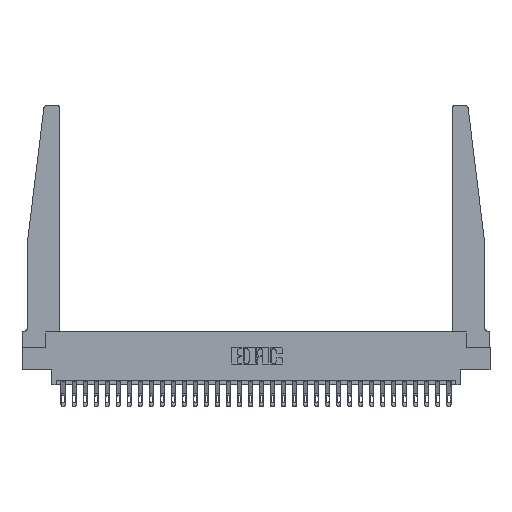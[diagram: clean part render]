
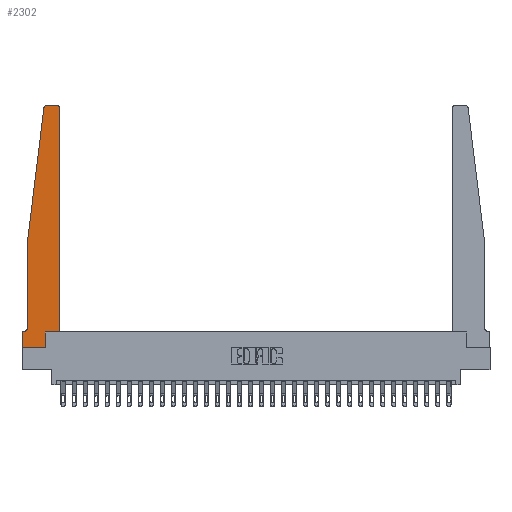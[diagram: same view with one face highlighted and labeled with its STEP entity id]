
A CAD part, top view. The second image highlights one B-rep face of the part: STEP entity #2302.
In plain terms, the highlighted planar face has unit normal (0, 0, 1).
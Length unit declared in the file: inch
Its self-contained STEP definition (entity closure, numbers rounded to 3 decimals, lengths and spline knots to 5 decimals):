
#673 = CARTESIAN_POINT ( 'NONE',  ( 0.24675, 2.72367, 0.37 ) ) ;
#2259 = CARTESIAN_POINT ( 'NONE',  ( 0.015, 0.2375, 0.37 ) ) ;
#2302 = ADVANCED_FACE ( 'NONE', ( #9067 ), #21267, .T. ) ;
#2728 = CARTESIAN_POINT ( 'NONE',  ( 0.425, 0.18, 0.37 ) ) ;
#3026 = LINE ( 'NONE', #15538, #26558 ) ;
#3067 = ORIENTED_EDGE ( 'NONE', *, *, #25364, .T. ) ;
#3499 = ORIENTED_EDGE ( 'NONE', *, *, #7070, .T. ) ;
#3506 = ORIENTED_EDGE ( 'NONE', *, *, #5088, .T. ) ;
#3825 = EDGE_CURVE ( 'NONE', #26339, #19652, #8687, .T. ) ;
#3912 = LINE ( 'NONE', #20043, #27462 ) ;
#4256 = CARTESIAN_POINT ( 'NONE',  ( 0., 0., 0.37 ) ) ;
#4514 = DIRECTION ( 'NONE',  ( -1., 0., 0. ) ) ;
#4518 = AXIS2_PLACEMENT_3D ( 'NONE', #7559, #23560, #9848 ) ;
#4815 = CARTESIAN_POINT ( 'NONE',  ( 0.065, 1.25, 0.37 ) ) ;
#4893 = VERTEX_POINT ( 'NONE', #23374 ) ;
#5088 = EDGE_CURVE ( 'NONE', #16684, #9863, #6162, .T. ) ;
#5407 = ORIENTED_EDGE ( 'NONE', *, *, #10375, .T. ) ;
#6162 = LINE ( 'NONE', #12579, #6842 ) ;
#6238 = ORIENTED_EDGE ( 'NONE', *, *, #28536, .T. ) ;
#6762 = CARTESIAN_POINT ( 'NONE',  ( 0.015, 0.1875, 0.37 ) ) ;
#6842 = VECTOR ( 'NONE', #28573, 39.37008 ) ;
#7034 = ORIENTED_EDGE ( 'NONE', *, *, #22006, .T. ) ;
#7070 = EDGE_CURVE ( 'NONE', #4893, #28127, #9926, .T. ) ;
#7249 = AXIS2_PLACEMENT_3D ( 'NONE', #2259, #18208, #4514 ) ;
#7559 = CARTESIAN_POINT ( 'NONE',  ( 0., 0.1875, 0.37 ) ) ;
#7808 = CIRCLE ( 'NONE', #23684, 0.03 ) ;
#8093 = LINE ( 'NONE', #21168, #25643 ) ;
#8476 = CARTESIAN_POINT ( 'NONE',  ( 0.425, 0.18, 0.37 ) ) ;
#8611 = DIRECTION ( 'NONE',  ( 1., 0., 0. ) ) ;
#8687 = LINE ( 'NONE', #12731, #13365 ) ;
#9067 = FACE_OUTER_BOUND ( 'NONE', #12613, .T. ) ;
#9848 = DIRECTION ( 'NONE',  ( 1., 0., 0. ) ) ;
#9863 = VERTEX_POINT ( 'NONE', #4256 ) ;
#9867 = CARTESIAN_POINT ( 'NONE',  ( 0.395, 2.75, 0.37 ) ) ;
#9926 = CIRCLE ( 'NONE', #7249, 0.05 ) ;
#10254 = CARTESIAN_POINT ( 'NONE',  ( 0.2605, 0., 0.37 ) ) ;
#10375 = EDGE_CURVE ( 'NONE', #21059, #12601, #27547, .T. ) ;
#10435 = EDGE_CURVE ( 'NONE', #19652, #23457, #13973, .T. ) ;
#10793 = DIRECTION ( 'NONE',  ( 0., 1., 0. ) ) ;
#12069 = DIRECTION ( 'NONE',  ( 0., -1., 0. ) ) ;
#12387 = DIRECTION ( 'NONE',  ( 0., 1., 0. ) ) ;
#12390 = LINE ( 'NONE', #16452, #23826 ) ;
#12539 = CARTESIAN_POINT ( 'NONE',  ( 0.395, 2.72, 0.37 ) ) ;
#12579 = CARTESIAN_POINT ( 'NONE',  ( 0., 0., 0.37 ) ) ;
#12601 = VERTEX_POINT ( 'NONE', #15994 ) ;
#12610 = CARTESIAN_POINT ( 'NONE',  ( 0.27653, 2.72, 0.37 ) ) ;
#12613 = EDGE_LOOP ( 'NONE', ( #5407, #28691, #7034, #3067, #3499, #14023, #3506, #6238, #23585, #26369, #19567, #15025 ) ) ;
#12731 = CARTESIAN_POINT ( 'NONE',  ( 0.425, 0.18, 0.37 ) ) ;
#13365 = VECTOR ( 'NONE', #24120, 39.37008 ) ;
#13423 = EDGE_CURVE ( 'NONE', #28127, #16684, #12390, .T. ) ;
#13764 = CARTESIAN_POINT ( 'NONE',  ( 0.425, 2.72, 0.37 ) ) ;
#13973 = LINE ( 'NONE', #8476, #25387 ) ;
#14023 = ORIENTED_EDGE ( 'NONE', *, *, #13423, .T. ) ;
#14846 = DIRECTION ( 'NONE',  ( 1., 0., 0. ) ) ;
#14914 = DIRECTION ( 'NONE',  ( 1., 0., 0. ) ) ;
#15025 = ORIENTED_EDGE ( 'NONE', *, *, #24142, .T. ) ;
#15538 = CARTESIAN_POINT ( 'NONE',  ( 0.065, 1.25, 0.37 ) ) ;
#15994 = CARTESIAN_POINT ( 'NONE',  ( 0.27653, 2.75, 0.37 ) ) ;
#16452 = CARTESIAN_POINT ( 'NONE',  ( 0.065, 0.1875, 0.37 ) ) ;
#16684 = VERTEX_POINT ( 'NONE', #28483 ) ;
#16929 = CARTESIAN_POINT ( 'NONE',  ( 0.2605, 0.18, 0.37 ) ) ;
#17380 = VECTOR ( 'NONE', #12387, 39.37008 ) ;
#17438 = CARTESIAN_POINT ( 'NONE',  ( 0.25, 2.75, 0.37 ) ) ;
#18179 = CIRCLE ( 'NONE', #23566, 0.03 ) ;
#18208 = DIRECTION ( 'NONE',  ( 0., 0., -1. ) ) ;
#19567 = ORIENTED_EDGE ( 'NONE', *, *, #10435, .T. ) ;
#19652 = VERTEX_POINT ( 'NONE', #2728 ) ;
#19717 = DIRECTION ( 'NONE',  ( -1., 0., 0. ) ) ;
#20043 = CARTESIAN_POINT ( 'NONE',  ( 0., 0., 0.37 ) ) ;
#20337 = VERTEX_POINT ( 'NONE', #673 ) ;
#21059 = VERTEX_POINT ( 'NONE', #9867 ) ;
#21168 = CARTESIAN_POINT ( 'NONE',  ( 0.065, 1.25, 0.37 ) ) ;
#21267 = PLANE ( 'NONE',  #4518 ) ;
#22006 = EDGE_CURVE ( 'NONE', #20337, #25275, #3026, .T. ) ;
#22194 = VECTOR ( 'NONE', #19717, 39.37008 ) ;
#23328 = DIRECTION ( 'NONE',  ( -1., 0., 0. ) ) ;
#23374 = CARTESIAN_POINT ( 'NONE',  ( 0.065, 0.2375, 0.37 ) ) ;
#23412 = LINE ( 'NONE', #16929, #17380 ) ;
#23457 = VERTEX_POINT ( 'NONE', #13764 ) ;
#23560 = DIRECTION ( 'NONE',  ( 0., 0., 1. ) ) ;
#23566 = AXIS2_PLACEMENT_3D ( 'NONE', #12610, #28599, #14914 ) ;
#23585 = ORIENTED_EDGE ( 'NONE', *, *, #27738, .T. ) ;
#23684 = AXIS2_PLACEMENT_3D ( 'NONE', #12539, #28538, #14846 ) ;
#23826 = VECTOR ( 'NONE', #23328, 39.37008 ) ;
#24120 = DIRECTION ( 'NONE',  ( 1., 0., 0. ) ) ;
#24142 = EDGE_CURVE ( 'NONE', #23457, #21059, #7808, .T. ) ;
#24705 = DIRECTION ( 'NONE',  ( -0.122, -0.992, 0. ) ) ;
#25275 = VERTEX_POINT ( 'NONE', #4815 ) ;
#25364 = EDGE_CURVE ( 'NONE', #25275, #4893, #8093, .T. ) ;
#25387 = VECTOR ( 'NONE', #10793, 39.37008 ) ;
#25643 = VECTOR ( 'NONE', #12069, 39.37008 ) ;
#26339 = VERTEX_POINT ( 'NONE', #29517 ) ;
#26369 = ORIENTED_EDGE ( 'NONE', *, *, #3825, .T. ) ;
#26558 = VECTOR ( 'NONE', #24705, 39.37008 ) ;
#27462 = VECTOR ( 'NONE', #8611, 39.37008 ) ;
#27547 = LINE ( 'NONE', #17438, #22194 ) ;
#27738 = EDGE_CURVE ( 'NONE', #27806, #26339, #23412, .T. ) ;
#27806 = VERTEX_POINT ( 'NONE', #10254 ) ;
#28127 = VERTEX_POINT ( 'NONE', #6762 ) ;
#28483 = CARTESIAN_POINT ( 'NONE',  ( 0., 0.1875, 0.37 ) ) ;
#28536 = EDGE_CURVE ( 'NONE', #9863, #27806, #3912, .T. ) ;
#28538 = DIRECTION ( 'NONE',  ( 0., 0., 1. ) ) ;
#28573 = DIRECTION ( 'NONE',  ( 0., -1., 0. ) ) ;
#28599 = DIRECTION ( 'NONE',  ( 0., 0., 1. ) ) ;
#28691 = ORIENTED_EDGE ( 'NONE', *, *, #28882, .T. ) ;
#28882 = EDGE_CURVE ( 'NONE', #12601, #20337, #18179, .T. ) ;
#29517 = CARTESIAN_POINT ( 'NONE',  ( 0.2605, 0.18, 0.37 ) ) ;
